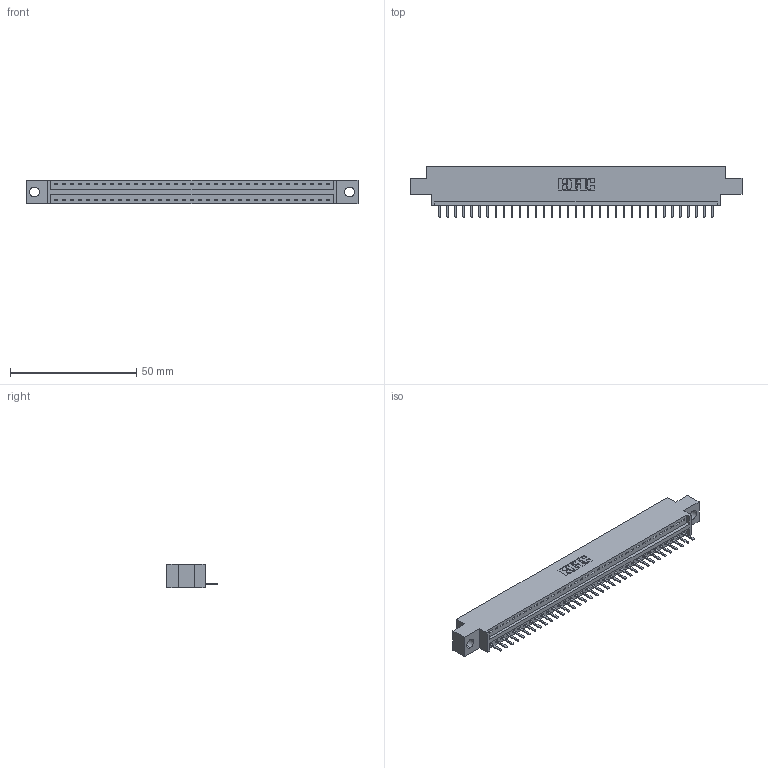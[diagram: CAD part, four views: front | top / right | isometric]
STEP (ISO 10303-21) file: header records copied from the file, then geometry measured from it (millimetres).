
FILE_DESCRIPTION (( 'STEP AP203' ), '1' );
FILE_NAME ('346-035-520-604.STEP', '2022-05-06T22:34:13', ( '' ), ( '' ), 'SwSTEP 2.0', 'SolidWorks 2020', '' );
FILE_SCHEMA (( 'CONFIG_CONTROL_DESIGN' ));
Length unit declared in the file: inch
Products named in the file (3): 345-292-001_345-293-120; 346 Part_0.170 Offset - 0.156 Dia-TH; 346-035-520-604
Assembly tree (36 placements, depth 2):
  346-035-520-604
    346 Part_0.170 Offset - 0.156 Dia-TH
    345-292-001_345-293-120  x35
Bounding box: 131.7 x 20.02 x 9.4 mm (x, y, z)
Volume: 12197 mm3; surface area: 14830.7 mm2
Topology: 36 solids, 36 shells, 2310 faces, 6817 edges, 4450 vertices
Faces by surface type: plane 1564, cylinder 746
Entity records: 23329 total; most frequent: CARTESIAN_POINT 4023, ORIENTED_EDGE 3978, DIRECTION 3543, EDGE_CURVE 1989, VECTOR 1713, LINE 1713, VERTEX_POINT 1322, AXIS2_PLACEMENT_3D 915
